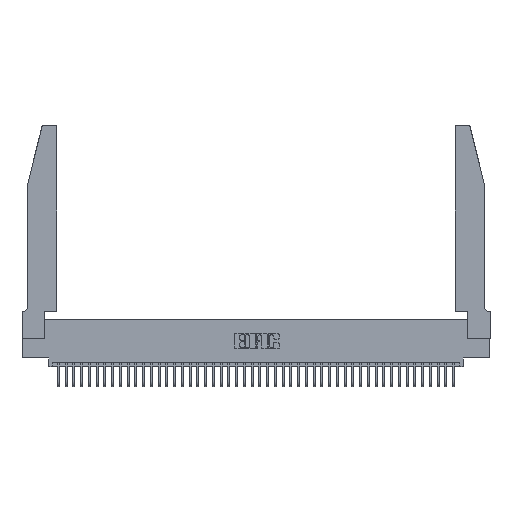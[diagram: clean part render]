
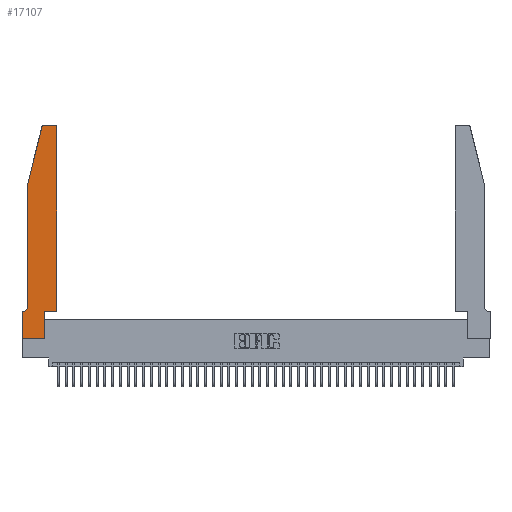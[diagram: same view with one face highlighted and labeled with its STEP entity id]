
A CAD part, top view. The second image highlights one B-rep face of the part: STEP entity #17107.
In plain terms, the highlighted planar face has unit normal (0, 0, 1).
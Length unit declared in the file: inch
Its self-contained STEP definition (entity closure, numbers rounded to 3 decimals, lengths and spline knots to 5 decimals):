
#384 = VECTOR ( 'NONE', #11069, 39.37008 ) ;
#537 = CARTESIAN_POINT ( 'NONE',  ( 0.2865, 0.35, 0.37 ) ) ;
#580 = AXIS2_PLACEMENT_3D ( 'NONE', #24229, #27965, #45341 ) ;
#1259 = EDGE_CURVE ( 'NONE', #40438, #37796, #17214, .T. ) ;
#1748 = DIRECTION ( 'NONE',  ( -1., 0., 0. ) ) ;
#1917 = CARTESIAN_POINT ( 'NONE',  ( 0., 0., 0.37 ) ) ;
#1943 = CARTESIAN_POINT ( 'NONE',  ( 0.284, 2.75, 0.37 ) ) ;
#3060 = VERTEX_POINT ( 'NONE', #14761 ) ;
#3275 = LINE ( 'NONE', #26614, #31694 ) ;
#3294 = VECTOR ( 'NONE', #7694, 39.37008 ) ;
#3307 = DIRECTION ( 'NONE',  ( 1., 0., 0. ) ) ;
#3352 = ORIENTED_EDGE ( 'NONE', *, *, #1259, .T. ) ;
#4055 = VERTEX_POINT ( 'NONE', #31472 ) ;
#4163 = CARTESIAN_POINT ( 'NONE',  ( 0., 0., 0.37 ) ) ;
#5252 = AXIS2_PLACEMENT_3D ( 'NONE', #37368, #16053, #44631 ) ;
#5411 = CARTESIAN_POINT ( 'NONE',  ( 0., 0.35, 0.37 ) ) ;
#5670 = AXIS2_PLACEMENT_3D ( 'NONE', #5411, #14167, #15784 ) ;
#6357 = ORIENTED_EDGE ( 'NONE', *, *, #14482, .T. ) ;
#6420 = AXIS2_PLACEMENT_3D ( 'NONE', #6743, #17642, #3307 ) ;
#6743 = CARTESIAN_POINT ( 'NONE',  ( 0.4205, 2.72, 0.37 ) ) ;
#7549 = CIRCLE ( 'NONE', #6420, 0.03 ) ;
#7694 = DIRECTION ( 'NONE',  ( 0., 1., 0. ) ) ;
#7867 = ORIENTED_EDGE ( 'NONE', *, *, #37526, .T. ) ;
#8701 = VERTEX_POINT ( 'NONE', #23645 ) ;
#8826 = DIRECTION ( 'NONE',  ( 0., -1., 0. ) ) ;
#10215 = CARTESIAN_POINT ( 'NONE',  ( 0.4505, 0.35, 0.37 ) ) ;
#10462 = LINE ( 'NONE', #27034, #41108 ) ;
#10626 = EDGE_CURVE ( 'NONE', #30543, #24553, #7549, .T. ) ;
#10682 = ORIENTED_EDGE ( 'NONE', *, *, #15641, .T. ) ;
#11069 = DIRECTION ( 'NONE',  ( 0., -1., 0. ) ) ;
#11088 = VERTEX_POINT ( 'NONE', #10215 ) ;
#11795 = CARTESIAN_POINT ( 'NONE',  ( 0.2865, 0.35, 0.37 ) ) ;
#12009 = CARTESIAN_POINT ( 'NONE',  ( 0.0755, 0.35, 0.37 ) ) ;
#12303 = CIRCLE ( 'NONE', #5252, 0.03 ) ;
#13330 = VERTEX_POINT ( 'NONE', #1943 ) ;
#14167 = DIRECTION ( 'NONE',  ( 0., 0., 1. ) ) ;
#14177 = DIRECTION ( 'NONE',  ( -0.239, -0.971, 0. ) ) ;
#14482 = EDGE_CURVE ( 'NONE', #8701, #4055, #26751, .T. ) ;
#14761 = CARTESIAN_POINT ( 'NONE',  ( 0., 0.35, 0.37 ) ) ;
#15641 = EDGE_CURVE ( 'NONE', #22842, #11088, #10462, .T. ) ;
#15784 = DIRECTION ( 'NONE',  ( 1., 0., 0. ) ) ;
#15909 = EDGE_CURVE ( 'NONE', #3060, #8701, #38307, .T. ) ;
#16053 = DIRECTION ( 'NONE',  ( 0., 0., 1. ) ) ;
#16796 = CARTESIAN_POINT ( 'NONE',  ( 0.4505, 0.35, 0.37 ) ) ;
#17004 = ORIENTED_EDGE ( 'NONE', *, *, #10626, .T. ) ;
#17107 = ADVANCED_FACE ( 'NONE', ( #41569 ), #44154, .T. ) ;
#17214 = LINE ( 'NONE', #21002, #33397 ) ;
#17642 = DIRECTION ( 'NONE',  ( 0., 0., 1. ) ) ;
#17955 = EDGE_CURVE ( 'NONE', #23527, #37131, #38716, .T. ) ;
#19817 = DIRECTION ( 'NONE',  ( 1., 0., 0. ) ) ;
#20195 = CARTESIAN_POINT ( 'NONE',  ( 0.4205, 2.75, 0.37 ) ) ;
#20335 = EDGE_CURVE ( 'NONE', #13330, #40438, #12303, .T. ) ;
#21002 = CARTESIAN_POINT ( 'NONE',  ( 0.0755, 2., 0.37 ) ) ;
#22842 = VERTEX_POINT ( 'NONE', #11795 ) ;
#23118 = LINE ( 'NONE', #12009, #42534 ) ;
#23378 = LINE ( 'NONE', #16796, #25011 ) ;
#23527 = VERTEX_POINT ( 'NONE', #38736 ) ;
#23645 = CARTESIAN_POINT ( 'NONE',  ( 0., 0., 0.37 ) ) ;
#24229 = CARTESIAN_POINT ( 'NONE',  ( 0.0055, 0.42, 0.37 ) ) ;
#24553 = VERTEX_POINT ( 'NONE', #20195 ) ;
#25011 = VECTOR ( 'NONE', #45209, 39.37008 ) ;
#26348 = CARTESIAN_POINT ( 'NONE',  ( 0.0055, 0.35, 0.37 ) ) ;
#26614 = CARTESIAN_POINT ( 'NONE',  ( 0.0755, 2., 0.37 ) ) ;
#26751 = LINE ( 'NONE', #1917, #32824 ) ;
#26960 = CARTESIAN_POINT ( 'NONE',  ( 0.4505, 2.72, 0.37 ) ) ;
#27034 = CARTESIAN_POINT ( 'NONE',  ( 0.4505, 0.35, 0.37 ) ) ;
#27965 = DIRECTION ( 'NONE',  ( 0., 0., -1. ) ) ;
#28848 = ORIENTED_EDGE ( 'NONE', *, *, #15909, .T. ) ;
#28921 = LINE ( 'NONE', #537, #3294 ) ;
#28975 = ORIENTED_EDGE ( 'NONE', *, *, #45960, .T. ) ;
#29290 = CARTESIAN_POINT ( 'NONE',  ( 0.25487, 2.72718, 0.37 ) ) ;
#30543 = VERTEX_POINT ( 'NONE', #26960 ) ;
#30595 = DIRECTION ( 'NONE',  ( 1., 0., 0. ) ) ;
#30758 = EDGE_LOOP ( 'NONE', ( #43027, #41477, #3352, #44005, #40250, #28975, #28848, #6357, #7867, #10682, #34150, #17004 ) ) ;
#31472 = CARTESIAN_POINT ( 'NONE',  ( 0.2865, 0., 0.37 ) ) ;
#31694 = VECTOR ( 'NONE', #8826, 39.37008 ) ;
#32824 = VECTOR ( 'NONE', #19817, 39.37008 ) ;
#33397 = VECTOR ( 'NONE', #14177, 39.37008 ) ;
#34150 = ORIENTED_EDGE ( 'NONE', *, *, #43338, .T. ) ;
#37131 = VERTEX_POINT ( 'NONE', #26348 ) ;
#37328 = CARTESIAN_POINT ( 'NONE',  ( 0.0755, 2., 0.37 ) ) ;
#37368 = CARTESIAN_POINT ( 'NONE',  ( 0.284, 2.72, 0.37 ) ) ;
#37526 = EDGE_CURVE ( 'NONE', #4055, #22842, #28921, .T. ) ;
#37796 = VERTEX_POINT ( 'NONE', #37328 ) ;
#38307 = LINE ( 'NONE', #4163, #384 ) ;
#38716 = CIRCLE ( 'NONE', #580, 0.07 ) ;
#38736 = CARTESIAN_POINT ( 'NONE',  ( 0.0755, 0.42, 0.37 ) ) ;
#38773 = VECTOR ( 'NONE', #45230, 39.37008 ) ;
#40250 = ORIENTED_EDGE ( 'NONE', *, *, #17955, .T. ) ;
#40438 = VERTEX_POINT ( 'NONE', #29290 ) ;
#41009 = LINE ( 'NONE', #41966, #38773 ) ;
#41108 = VECTOR ( 'NONE', #30595, 39.37008 ) ;
#41477 = ORIENTED_EDGE ( 'NONE', *, *, #20335, .T. ) ;
#41569 = FACE_OUTER_BOUND ( 'NONE', #30758, .T. ) ;
#41966 = CARTESIAN_POINT ( 'NONE',  ( 0.2605, 2.75, 0.37 ) ) ;
#42534 = VECTOR ( 'NONE', #1748, 39.37008 ) ;
#43027 = ORIENTED_EDGE ( 'NONE', *, *, #44851, .T. ) ;
#43146 = EDGE_CURVE ( 'NONE', #37796, #23527, #3275, .T. ) ;
#43338 = EDGE_CURVE ( 'NONE', #11088, #30543, #23378, .T. ) ;
#44005 = ORIENTED_EDGE ( 'NONE', *, *, #43146, .T. ) ;
#44154 = PLANE ( 'NONE',  #5670 ) ;
#44631 = DIRECTION ( 'NONE',  ( 1., 0., 0. ) ) ;
#44851 = EDGE_CURVE ( 'NONE', #24553, #13330, #41009, .T. ) ;
#45209 = DIRECTION ( 'NONE',  ( 0., 1., 0. ) ) ;
#45230 = DIRECTION ( 'NONE',  ( -1., 0., 0. ) ) ;
#45341 = DIRECTION ( 'NONE',  ( -1., 0., 0. ) ) ;
#45960 = EDGE_CURVE ( 'NONE', #37131, #3060, #23118, .T. ) ;
